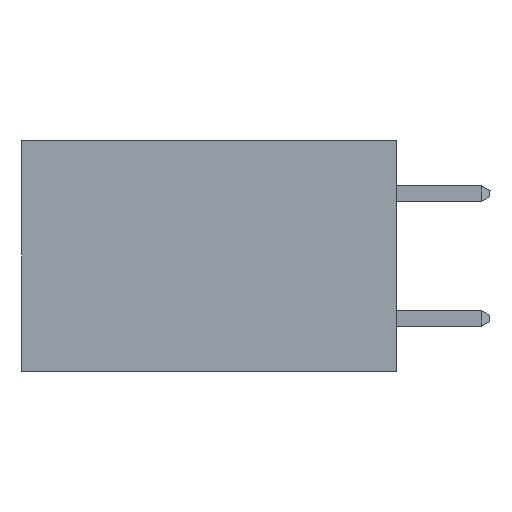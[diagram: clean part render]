
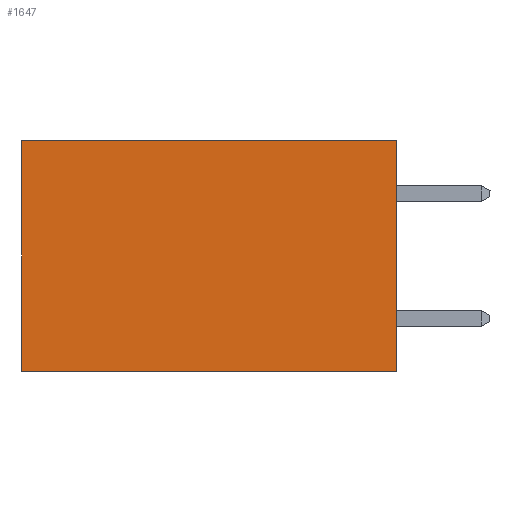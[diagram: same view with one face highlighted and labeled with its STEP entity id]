
A CAD part, left-side view. The second image highlights one B-rep face of the part: STEP entity #1647.
In plain terms, the highlighted planar face has unit normal (-1, 0, 0).
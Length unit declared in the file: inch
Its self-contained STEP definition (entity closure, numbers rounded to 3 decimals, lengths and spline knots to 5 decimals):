
#868 = FACE_OUTER_BOUND ( 'NONE', #4595, .T. ) ;
#1647 = ADVANCED_FACE ( 'NONE', ( #868 ), #8018, .F. ) ;
#1672 = LINE ( 'NONE', #11641, #8777 ) ;
#1683 = VECTOR ( 'NONE', #11951, 39.37008 ) ;
#2653 = CARTESIAN_POINT ( 'NONE',  ( 0.298, 0., -0.37 ) ) ;
#2668 = LINE ( 'NONE', #7023, #18132 ) ;
#4121 = DIRECTION ( 'NONE',  ( 0., 0., -1. ) ) ;
#4595 = EDGE_LOOP ( 'NONE', ( #10906, #4899, #10550, #10052 ) ) ;
#4899 = ORIENTED_EDGE ( 'NONE', *, *, #17499, .F. ) ;
#5652 = DIRECTION ( 'NONE',  ( 0., 0., -1. ) ) ;
#6830 = CARTESIAN_POINT ( 'NONE',  ( 0.298, 0., 0. ) ) ;
#7023 = CARTESIAN_POINT ( 'NONE',  ( 0.298, 0.6, 0. ) ) ;
#7178 = EDGE_CURVE ( 'NONE', #15069, #14648, #18126, .T. ) ;
#8018 = PLANE ( 'NONE',  #13372 ) ;
#8034 = EDGE_CURVE ( 'NONE', #14648, #12941, #2668, .T. ) ;
#8271 = LINE ( 'NONE', #15060, #16240 ) ;
#8777 = VECTOR ( 'NONE', #4121, 39.37008 ) ;
#9640 = CARTESIAN_POINT ( 'NONE',  ( 0.298, 0.6, -0.37 ) ) ;
#10052 = ORIENTED_EDGE ( 'NONE', *, *, #7178, .T. ) ;
#10550 = ORIENTED_EDGE ( 'NONE', *, *, #16584, .F. ) ;
#10906 = ORIENTED_EDGE ( 'NONE', *, *, #8034, .T. ) ;
#11641 = CARTESIAN_POINT ( 'NONE',  ( 0.298, 0., 0. ) ) ;
#11951 = DIRECTION ( 'NONE',  ( 0., 1., 0. ) ) ;
#12374 = DIRECTION ( 'NONE',  ( 0., 0., -1. ) ) ;
#12941 = VERTEX_POINT ( 'NONE', #9640 ) ;
#13372 = AXIS2_PLACEMENT_3D ( 'NONE', #6830, #19276, #12374 ) ;
#14648 = VERTEX_POINT ( 'NONE', #15229 ) ;
#15060 = CARTESIAN_POINT ( 'NONE',  ( 0.298, 0., -0.37 ) ) ;
#15069 = VERTEX_POINT ( 'NONE', #16978 ) ;
#15229 = CARTESIAN_POINT ( 'NONE',  ( 0.298, 0.6, 0. ) ) ;
#15367 = VERTEX_POINT ( 'NONE', #2653 ) ;
#16151 = CARTESIAN_POINT ( 'NONE',  ( 0.298, 0., 0. ) ) ;
#16240 = VECTOR ( 'NONE', #16567, 39.37008 ) ;
#16567 = DIRECTION ( 'NONE',  ( 0., 1., 0. ) ) ;
#16584 = EDGE_CURVE ( 'NONE', #15069, #15367, #1672, .T. ) ;
#16978 = CARTESIAN_POINT ( 'NONE',  ( 0.298, 0., 0. ) ) ;
#17499 = EDGE_CURVE ( 'NONE', #15367, #12941, #8271, .T. ) ;
#18126 = LINE ( 'NONE', #16151, #1683 ) ;
#18132 = VECTOR ( 'NONE', #5652, 39.37008 ) ;
#19276 = DIRECTION ( 'NONE',  ( 1., 0., 0. ) ) ;
